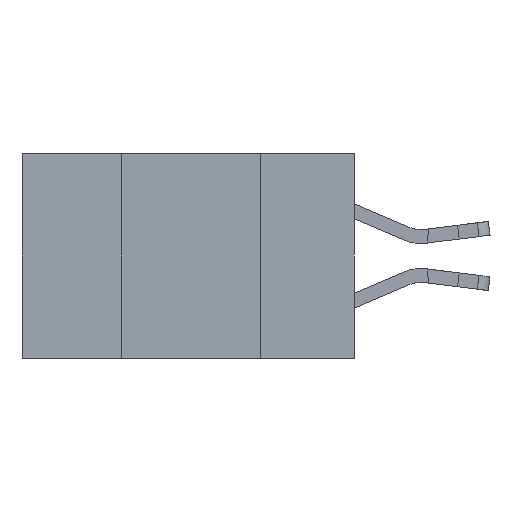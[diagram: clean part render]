
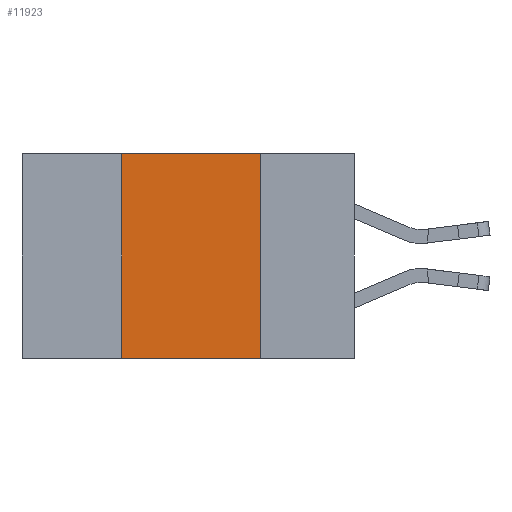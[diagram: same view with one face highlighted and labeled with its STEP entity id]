
A CAD part, left-side view. The second image highlights one B-rep face of the part: STEP entity #11923.
In plain terms, the highlighted planar face has unit normal (-1, 0, 0).
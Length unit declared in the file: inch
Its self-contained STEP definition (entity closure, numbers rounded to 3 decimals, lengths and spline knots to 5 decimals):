
#1960 = LINE ( 'NONE', #9471, #11402 ) ;
#2765 = EDGE_CURVE ( 'NONE', #2837, #8581, #2920, .T. ) ;
#2837 = VERTEX_POINT ( 'NONE', #5999 ) ;
#2920 = LINE ( 'NONE', #5059, #13517 ) ;
#3201 = VECTOR ( 'NONE', #12494, 39.37008 ) ;
#4023 = FACE_OUTER_BOUND ( 'NONE', #11616, .T. ) ;
#4097 = LINE ( 'NONE', #11512, #3201 ) ;
#4701 = CARTESIAN_POINT ( 'NONE',  ( 0., 0.17, -0.37 ) ) ;
#4798 = EDGE_CURVE ( 'NONE', #10535, #5134, #7537, .T. ) ;
#5046 = AXIS2_PLACEMENT_3D ( 'NONE', #10216, #11380, #8217 ) ;
#5059 = CARTESIAN_POINT ( 'NONE',  ( 0., 0.17, -0.37 ) ) ;
#5127 = DIRECTION ( 'NONE',  ( 0., 0., -1. ) ) ;
#5134 = VERTEX_POINT ( 'NONE', #9152 ) ;
#5421 = CARTESIAN_POINT ( 'NONE',  ( 0., 0.42, -0.37 ) ) ;
#5999 = CARTESIAN_POINT ( 'NONE',  ( 0., 0.17, 0. ) ) ;
#6282 = DIRECTION ( 'NONE',  ( 0., -1., 0. ) ) ;
#6607 = EDGE_CURVE ( 'NONE', #10535, #8581, #4097, .T. ) ;
#7099 = CARTESIAN_POINT ( 'NONE',  ( 0., 0.42, -0.37 ) ) ;
#7537 = LINE ( 'NONE', #5421, #13072 ) ;
#8217 = DIRECTION ( 'NONE',  ( 0., 0., -1. ) ) ;
#8581 = VERTEX_POINT ( 'NONE', #4701 ) ;
#8834 = ORIENTED_EDGE ( 'NONE', *, *, #4798, .F. ) ;
#9152 = CARTESIAN_POINT ( 'NONE',  ( 0., 0.42, 0. ) ) ;
#9471 = CARTESIAN_POINT ( 'NONE',  ( 0., 0.6, 0. ) ) ;
#9634 = DIRECTION ( 'NONE',  ( 0., 0., 1. ) ) ;
#10055 = EDGE_CURVE ( 'NONE', #5134, #2837, #1960, .T. ) ;
#10216 = CARTESIAN_POINT ( 'NONE',  ( 0., 0.6, 0. ) ) ;
#10325 = ORIENTED_EDGE ( 'NONE', *, *, #10055, .F. ) ;
#10535 = VERTEX_POINT ( 'NONE', #7099 ) ;
#11380 = DIRECTION ( 'NONE',  ( 1., 0., 0. ) ) ;
#11402 = VECTOR ( 'NONE', #6282, 39.37008 ) ;
#11446 = PLANE ( 'NONE',  #5046 ) ;
#11512 = CARTESIAN_POINT ( 'NONE',  ( 0., 0.6, -0.37 ) ) ;
#11616 = EDGE_LOOP ( 'NONE', ( #12485, #10325, #8834, #12206 ) ) ;
#11923 = ADVANCED_FACE ( 'NONE', ( #4023 ), #11446, .F. ) ;
#12206 = ORIENTED_EDGE ( 'NONE', *, *, #6607, .T. ) ;
#12485 = ORIENTED_EDGE ( 'NONE', *, *, #2765, .F. ) ;
#12494 = DIRECTION ( 'NONE',  ( 0., -1., 0. ) ) ;
#13072 = VECTOR ( 'NONE', #9634, 39.37008 ) ;
#13517 = VECTOR ( 'NONE', #5127, 39.37008 ) ;
